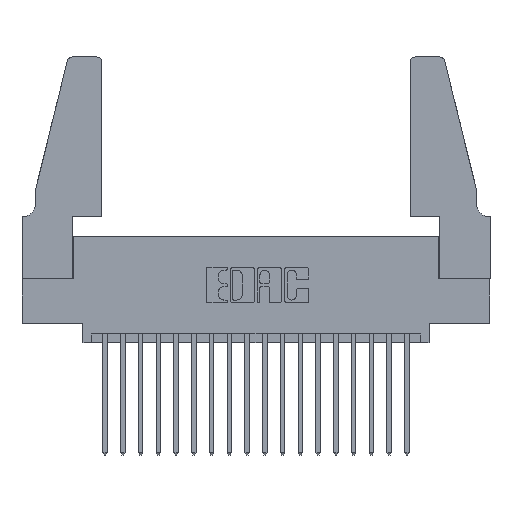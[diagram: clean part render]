
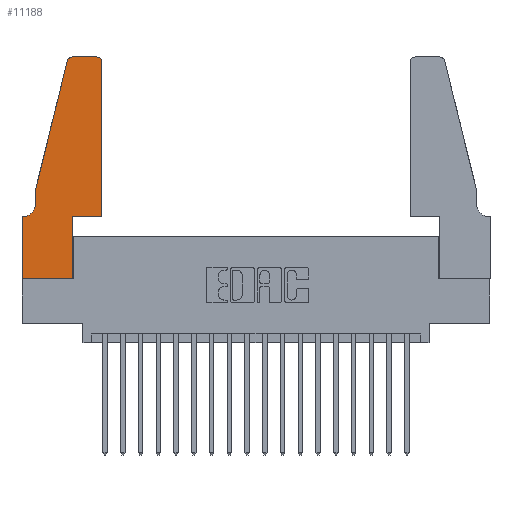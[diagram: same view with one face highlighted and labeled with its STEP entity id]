
A CAD part, top view. The second image highlights one B-rep face of the part: STEP entity #11188.
In plain terms, the highlighted planar face has unit normal (0, 0, 1).
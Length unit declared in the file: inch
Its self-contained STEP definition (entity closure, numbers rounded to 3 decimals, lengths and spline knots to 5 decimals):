
#153 = LINE ( 'NONE', #8300, #19380 ) ;
#225 = DIRECTION ( 'NONE',  ( 0., 0., -1. ) ) ;
#476 = EDGE_CURVE ( 'NONE', #17574, #11732, #8479, .T. ) ;
#635 = VECTOR ( 'NONE', #7144, 39.37008 ) ;
#933 = VECTOR ( 'NONE', #15025, 39.37008 ) ;
#1316 = VECTOR ( 'NONE', #12493, 39.37008 ) ;
#1625 = VERTEX_POINT ( 'NONE', #13856 ) ;
#1633 = ORIENTED_EDGE ( 'NONE', *, *, #9396, .T. ) ;
#1801 = VERTEX_POINT ( 'NONE', #7573 ) ;
#1806 = LINE ( 'NONE', #9068, #5874 ) ;
#1886 = AXIS2_PLACEMENT_3D ( 'NONE', #2971, #13478, #4499 ) ;
#2462 = CARTESIAN_POINT ( 'NONE',  ( 0.4505, 0.35, 0.37 ) ) ;
#2557 = EDGE_CURVE ( 'NONE', #6705, #5094, #153, .T. ) ;
#2711 = EDGE_LOOP ( 'NONE', ( #14252, #16116, #8880, #7765, #16884, #5415, #10052, #15273, #14777, #7517, #12937, #1633 ) ) ;
#2937 = CARTESIAN_POINT ( 'NONE',  ( 0.4505, 0.35, 0.37 ) ) ;
#2971 = CARTESIAN_POINT ( 'NONE',  ( 0.284, 1.22, 0.37 ) ) ;
#3185 = EDGE_CURVE ( 'NONE', #4165, #10892, #12918, .T. ) ;
#3239 = EDGE_CURVE ( 'NONE', #10892, #17373, #19117, .T. ) ;
#3417 = CIRCLE ( 'NONE', #7914, 0.07 ) ;
#3466 = VECTOR ( 'NONE', #7473, 39.37008 ) ;
#3503 = EDGE_CURVE ( 'NONE', #9627, #13102, #1806, .T. ) ;
#3660 = DIRECTION ( 'NONE',  ( 1., 0., 0. ) ) ;
#4009 = EDGE_CURVE ( 'NONE', #11732, #9627, #15499, .T. ) ;
#4011 = EDGE_CURVE ( 'NONE', #5094, #1801, #7487, .T. ) ;
#4165 = VERTEX_POINT ( 'NONE', #15295 ) ;
#4266 = CARTESIAN_POINT ( 'NONE',  ( 0.0755, 0.35, 0.37 ) ) ;
#4432 = CARTESIAN_POINT ( 'NONE',  ( 0., 0., 0.37 ) ) ;
#4440 = DIRECTION ( 'NONE',  ( -1., 0., 0. ) ) ;
#4499 = DIRECTION ( 'NONE',  ( 1., 0., 0. ) ) ;
#5094 = VERTEX_POINT ( 'NONE', #6908 ) ;
#5397 = LINE ( 'NONE', #11028, #1316 ) ;
#5415 = ORIENTED_EDGE ( 'NONE', *, *, #476, .T. ) ;
#5666 = AXIS2_PLACEMENT_3D ( 'NONE', #17717, #8667, #19257 ) ;
#5874 = VECTOR ( 'NONE', #16598, 39.37008 ) ;
#6705 = VERTEX_POINT ( 'NONE', #16366 ) ;
#6908 = CARTESIAN_POINT ( 'NONE',  ( 0.284, 1.25, 0.37 ) ) ;
#7144 = DIRECTION ( 'NONE',  ( -0.239, -0.971, 0. ) ) ;
#7473 = DIRECTION ( 'NONE',  ( 0., -1., 0. ) ) ;
#7487 = CIRCLE ( 'NONE', #1886, 0.03 ) ;
#7517 = ORIENTED_EDGE ( 'NONE', *, *, #3185, .T. ) ;
#7573 = CARTESIAN_POINT ( 'NONE',  ( 0.25487, 1.22718, 0.37 ) ) ;
#7578 = EDGE_CURVE ( 'NONE', #1625, #17574, #3417, .T. ) ;
#7765 = ORIENTED_EDGE ( 'NONE', *, *, #16694, .T. ) ;
#7858 = DIRECTION ( 'NONE',  ( -1., 0., 0. ) ) ;
#7914 = AXIS2_PLACEMENT_3D ( 'NONE', #9366, #225, #10884 ) ;
#8097 = DIRECTION ( 'NONE',  ( 1., 0., 0. ) ) ;
#8163 = PLANE ( 'NONE',  #14647 ) ;
#8300 = CARTESIAN_POINT ( 'NONE',  ( 0.2605, 1.25, 0.37 ) ) ;
#8469 = VECTOR ( 'NONE', #8097, 39.37008 ) ;
#8479 = LINE ( 'NONE', #4266, #16025 ) ;
#8667 = DIRECTION ( 'NONE',  ( 0., 0., 1. ) ) ;
#8880 = ORIENTED_EDGE ( 'NONE', *, *, #15588, .T. ) ;
#8976 = CARTESIAN_POINT ( 'NONE',  ( 0.2865, 0.35, 0.37 ) ) ;
#9068 = CARTESIAN_POINT ( 'NONE',  ( 0., 0., 0.37 ) ) ;
#9366 = CARTESIAN_POINT ( 'NONE',  ( 0.0055, 0.42, 0.37 ) ) ;
#9396 = EDGE_CURVE ( 'NONE', #17373, #6705, #15855, .T. ) ;
#9543 = CARTESIAN_POINT ( 'NONE',  ( 0.4505, 0.35, 0.37 ) ) ;
#9627 = VERTEX_POINT ( 'NONE', #12224 ) ;
#10052 = ORIENTED_EDGE ( 'NONE', *, *, #4009, .T. ) ;
#10236 = EDGE_CURVE ( 'NONE', #13102, #4165, #13447, .T. ) ;
#10344 = CARTESIAN_POINT ( 'NONE',  ( 0.0055, 0.35, 0.37 ) ) ;
#10884 = DIRECTION ( 'NONE',  ( -1., 0., 0. ) ) ;
#10892 = VERTEX_POINT ( 'NONE', #2937 ) ;
#11028 = CARTESIAN_POINT ( 'NONE',  ( 0.0755, 0.5, 0.37 ) ) ;
#11188 = ADVANCED_FACE ( 'NONE', ( #17010 ), #8163, .T. ) ;
#11218 = CARTESIAN_POINT ( 'NONE',  ( 0., 0.35, 0.37 ) ) ;
#11387 = CARTESIAN_POINT ( 'NONE',  ( 0.4505, 1.22, 0.37 ) ) ;
#11732 = VERTEX_POINT ( 'NONE', #15371 ) ;
#12224 = CARTESIAN_POINT ( 'NONE',  ( 0., 0., 0.37 ) ) ;
#12493 = DIRECTION ( 'NONE',  ( 0., -1., 0. ) ) ;
#12676 = DIRECTION ( 'NONE',  ( 0., 0., 1. ) ) ;
#12706 = LINE ( 'NONE', #13099, #635 ) ;
#12918 = LINE ( 'NONE', #2462, #8469 ) ;
#12937 = ORIENTED_EDGE ( 'NONE', *, *, #3239, .T. ) ;
#13099 = CARTESIAN_POINT ( 'NONE',  ( 0.0755, 0.5, 0.37 ) ) ;
#13102 = VERTEX_POINT ( 'NONE', #13153 ) ;
#13153 = CARTESIAN_POINT ( 'NONE',  ( 0.2865, 0., 0.37 ) ) ;
#13447 = LINE ( 'NONE', #8976, #933 ) ;
#13478 = DIRECTION ( 'NONE',  ( 0., 0., 1. ) ) ;
#13618 = DIRECTION ( 'NONE',  ( 0., 1., 0. ) ) ;
#13856 = CARTESIAN_POINT ( 'NONE',  ( 0.0755, 0.42, 0.37 ) ) ;
#14252 = ORIENTED_EDGE ( 'NONE', *, *, #2557, .T. ) ;
#14647 = AXIS2_PLACEMENT_3D ( 'NONE', #11218, #12676, #3660 ) ;
#14777 = ORIENTED_EDGE ( 'NONE', *, *, #10236, .T. ) ;
#15025 = DIRECTION ( 'NONE',  ( 0., 1., 0. ) ) ;
#15054 = VECTOR ( 'NONE', #13618, 39.37008 ) ;
#15273 = ORIENTED_EDGE ( 'NONE', *, *, #3503, .T. ) ;
#15295 = CARTESIAN_POINT ( 'NONE',  ( 0.2865, 0.35, 0.37 ) ) ;
#15371 = CARTESIAN_POINT ( 'NONE',  ( 0., 0.35, 0.37 ) ) ;
#15499 = LINE ( 'NONE', #4432, #3466 ) ;
#15567 = CARTESIAN_POINT ( 'NONE',  ( 0.0755, 0.5, 0.37 ) ) ;
#15588 = EDGE_CURVE ( 'NONE', #1801, #16004, #12706, .T. ) ;
#15855 = CIRCLE ( 'NONE', #5666, 0.03 ) ;
#16004 = VERTEX_POINT ( 'NONE', #15567 ) ;
#16025 = VECTOR ( 'NONE', #7858, 39.37008 ) ;
#16116 = ORIENTED_EDGE ( 'NONE', *, *, #4011, .T. ) ;
#16366 = CARTESIAN_POINT ( 'NONE',  ( 0.4205, 1.25, 0.37 ) ) ;
#16598 = DIRECTION ( 'NONE',  ( 1., 0., 0. ) ) ;
#16694 = EDGE_CURVE ( 'NONE', #16004, #1625, #5397, .T. ) ;
#16884 = ORIENTED_EDGE ( 'NONE', *, *, #7578, .T. ) ;
#17010 = FACE_OUTER_BOUND ( 'NONE', #2711, .T. ) ;
#17373 = VERTEX_POINT ( 'NONE', #11387 ) ;
#17574 = VERTEX_POINT ( 'NONE', #10344 ) ;
#17717 = CARTESIAN_POINT ( 'NONE',  ( 0.4205, 1.22, 0.37 ) ) ;
#19117 = LINE ( 'NONE', #9543, #15054 ) ;
#19257 = DIRECTION ( 'NONE',  ( 1., 0., 0. ) ) ;
#19380 = VECTOR ( 'NONE', #4440, 39.37008 ) ;
